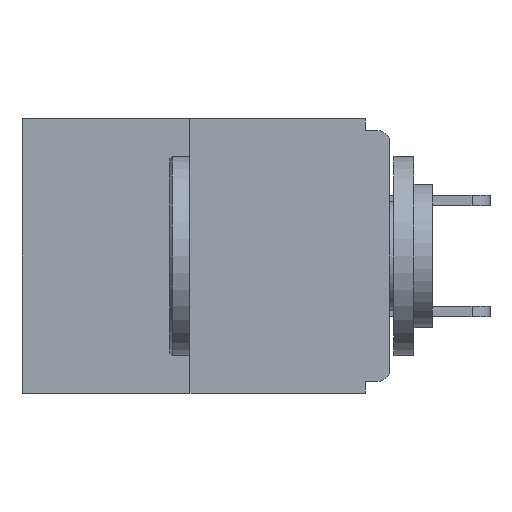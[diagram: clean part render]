
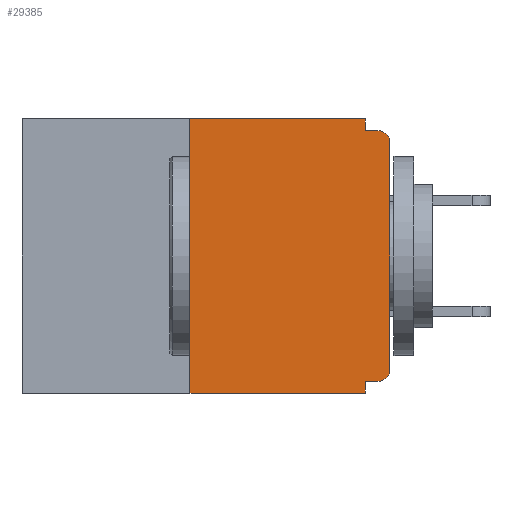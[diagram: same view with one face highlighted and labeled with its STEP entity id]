
A CAD part, left-side view. The second image highlights one B-rep face of the part: STEP entity #29385.
In plain terms, the highlighted planar face has unit normal (-1, 0, 0).
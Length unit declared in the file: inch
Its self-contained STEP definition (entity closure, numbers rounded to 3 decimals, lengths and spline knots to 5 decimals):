
#14 = VERTEX_POINT ( 'NONE', #25178 ) ;
#352 = EDGE_CURVE ( 'NONE', #3660, #29064, #7460, .T. ) ;
#362 = DIRECTION ( 'NONE',  ( -1., 0., 0. ) ) ;
#562 = ORIENTED_EDGE ( 'NONE', *, *, #352, .F. ) ;
#600 = DIRECTION ( 'NONE',  ( 0., 0., -1. ) ) ;
#638 = EDGE_CURVE ( 'NONE', #11287, #21774, #6324, .T. ) ;
#1334 = DIRECTION ( 'NONE',  ( 0., 0., -1. ) ) ;
#2084 = DIRECTION ( 'NONE',  ( -1., 0., 0. ) ) ;
#2227 = EDGE_CURVE ( 'NONE', #29064, #6849, #28361, .T. ) ;
#2376 = VECTOR ( 'NONE', #9399, 39.37008 ) ;
#2512 = AXIS2_PLACEMENT_3D ( 'NONE', #16419, #2084, #18838 ) ;
#3335 = LINE ( 'NONE', #15566, #28095 ) ;
#3660 = VERTEX_POINT ( 'NONE', #17078 ) ;
#4102 = ORIENTED_EDGE ( 'NONE', *, *, #24748, .T. ) ;
#5498 = CARTESIAN_POINT ( 'NONE',  ( 0., 0.031, -0.343 ) ) ;
#5531 = CARTESIAN_POINT ( 'NONE',  ( 0., 0., -0.313 ) ) ;
#6081 = CARTESIAN_POINT ( 'NONE',  ( 0., 0.015, -0.015 ) ) ;
#6324 = CIRCLE ( 'NONE', #2512, 0.015 ) ;
#6634 = ORIENTED_EDGE ( 'NONE', *, *, #23207, .F. ) ;
#6849 = VERTEX_POINT ( 'NONE', #26434 ) ;
#6910 = EDGE_CURVE ( 'NONE', #9059, #3660, #30504, .T. ) ;
#6937 = ORIENTED_EDGE ( 'NONE', *, *, #2227, .F. ) ;
#7325 = VECTOR ( 'NONE', #19549, 39.37008 ) ;
#7460 = LINE ( 'NONE', #26230, #19457 ) ;
#7573 = CARTESIAN_POINT ( 'NONE',  ( 0., 0.031, 0. ) ) ;
#8183 = LINE ( 'NONE', #5498, #24750 ) ;
#8308 = CARTESIAN_POINT ( 'NONE',  ( 0., 0.46, -0.343 ) ) ;
#8681 = EDGE_LOOP ( 'NONE', ( #562, #26648, #9382, #23236, #6634, #16982, #4102, #14969, #30752, #6937 ) ) ;
#9059 = VERTEX_POINT ( 'NONE', #20648 ) ;
#9098 = DIRECTION ( 'NONE',  ( 0., -1., 0. ) ) ;
#9382 = ORIENTED_EDGE ( 'NONE', *, *, #13077, .T. ) ;
#9399 = DIRECTION ( 'NONE',  ( 0., 0., 1. ) ) ;
#10451 = VERTEX_POINT ( 'NONE', #13067 ) ;
#11226 = VECTOR ( 'NONE', #22491, 39.37008 ) ;
#11287 = VERTEX_POINT ( 'NONE', #24417 ) ;
#12739 = LINE ( 'NONE', #22858, #16511 ) ;
#13067 = CARTESIAN_POINT ( 'NONE',  ( 0., 0.015, -0.328 ) ) ;
#13077 = EDGE_CURVE ( 'NONE', #9059, #21315, #27804, .T. ) ;
#13222 = DIRECTION ( 'NONE',  ( 1., 0., 0. ) ) ;
#13752 = CARTESIAN_POINT ( 'NONE',  ( 0., 0.031, 0. ) ) ;
#14644 = CARTESIAN_POINT ( 'NONE',  ( 0., 0.015, -0.313 ) ) ;
#14969 = ORIENTED_EDGE ( 'NONE', *, *, #638, .T. ) ;
#15566 = CARTESIAN_POINT ( 'NONE',  ( 0., 0., 0. ) ) ;
#15785 = DIRECTION ( 'NONE',  ( 0., 1., 0. ) ) ;
#16419 = CARTESIAN_POINT ( 'NONE',  ( 0., 0.015, -0.03 ) ) ;
#16492 = DIRECTION ( 'NONE',  ( 0., 0., -1. ) ) ;
#16511 = VECTOR ( 'NONE', #15785, 39.37008 ) ;
#16982 = ORIENTED_EDGE ( 'NONE', *, *, #30364, .T. ) ;
#17078 = CARTESIAN_POINT ( 'NONE',  ( 0., 0.25, 0. ) ) ;
#17099 = DIRECTION ( 'NONE',  ( 0., 0., -1. ) ) ;
#17329 = CARTESIAN_POINT ( 'NONE',  ( 0., 0., -0.015 ) ) ;
#18292 = AXIS2_PLACEMENT_3D ( 'NONE', #30374, #13222, #1334 ) ;
#18838 = DIRECTION ( 'NONE',  ( 0., 0., -1. ) ) ;
#19457 = VECTOR ( 'NONE', #9098, 39.37008 ) ;
#19517 = EDGE_CURVE ( 'NONE', #14, #21315, #8183, .T. ) ;
#19549 = DIRECTION ( 'NONE',  ( 0., -1., 0. ) ) ;
#20648 = CARTESIAN_POINT ( 'NONE',  ( 0., 0.25, -0.343 ) ) ;
#21204 = CIRCLE ( 'NONE', #30565, 0.015 ) ;
#21315 = VERTEX_POINT ( 'NONE', #29384 ) ;
#21510 = EDGE_CURVE ( 'NONE', #6849, #21774, #23084, .T. ) ;
#21578 = VECTOR ( 'NONE', #16492, 39.37008 ) ;
#21658 = FACE_OUTER_BOUND ( 'NONE', #8681, .T. ) ;
#21704 = CARTESIAN_POINT ( 'NONE',  ( 0., 0.25, 0. ) ) ;
#21774 = VERTEX_POINT ( 'NONE', #6081 ) ;
#22491 = DIRECTION ( 'NONE',  ( 0., -1., 0. ) ) ;
#22858 = CARTESIAN_POINT ( 'NONE',  ( 0., 0., -0.328 ) ) ;
#23084 = LINE ( 'NONE', #17329, #7325 ) ;
#23207 = EDGE_CURVE ( 'NONE', #10451, #14, #12739, .T. ) ;
#23236 = ORIENTED_EDGE ( 'NONE', *, *, #19517, .F. ) ;
#24417 = CARTESIAN_POINT ( 'NONE',  ( 0., 0., -0.03 ) ) ;
#24748 = EDGE_CURVE ( 'NONE', #29216, #11287, #3335, .T. ) ;
#24750 = VECTOR ( 'NONE', #600, 39.37008 ) ;
#25178 = CARTESIAN_POINT ( 'NONE',  ( 0., 0.031, -0.328 ) ) ;
#26230 = CARTESIAN_POINT ( 'NONE',  ( 0., 0.46, 0. ) ) ;
#26434 = CARTESIAN_POINT ( 'NONE',  ( 0., 0.031, -0.015 ) ) ;
#26648 = ORIENTED_EDGE ( 'NONE', *, *, #6910, .F. ) ;
#27646 = PLANE ( 'NONE',  #18292 ) ;
#27804 = LINE ( 'NONE', #8308, #11226 ) ;
#28095 = VECTOR ( 'NONE', #29882, 39.37008 ) ;
#28361 = LINE ( 'NONE', #13752, #21578 ) ;
#29064 = VERTEX_POINT ( 'NONE', #7573 ) ;
#29216 = VERTEX_POINT ( 'NONE', #5531 ) ;
#29384 = CARTESIAN_POINT ( 'NONE',  ( 0., 0.031, -0.343 ) ) ;
#29385 = ADVANCED_FACE ( 'NONE', ( #21658 ), #27646, .F. ) ;
#29882 = DIRECTION ( 'NONE',  ( 0., 0., 1. ) ) ;
#30364 = EDGE_CURVE ( 'NONE', #10451, #29216, #21204, .T. ) ;
#30374 = CARTESIAN_POINT ( 'NONE',  ( 0., 0.46, 0. ) ) ;
#30504 = LINE ( 'NONE', #21704, #2376 ) ;
#30565 = AXIS2_PLACEMENT_3D ( 'NONE', #14644, #362, #17099 ) ;
#30752 = ORIENTED_EDGE ( 'NONE', *, *, #21510, .F. ) ;
